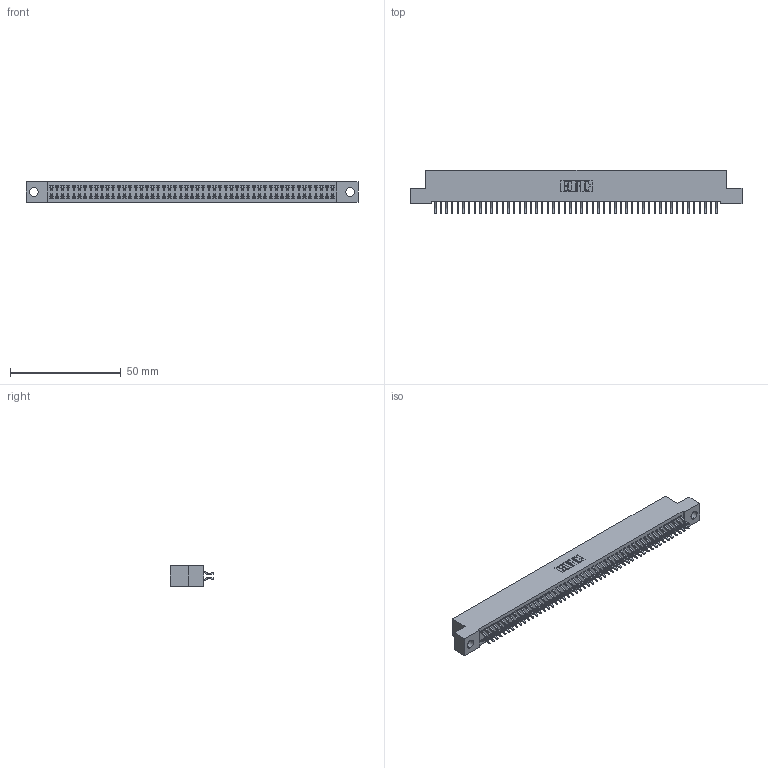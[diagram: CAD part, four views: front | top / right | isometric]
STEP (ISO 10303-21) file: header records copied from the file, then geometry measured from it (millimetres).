
FILE_DESCRIPTION (( 'STEP AP203' ), '1' );
FILE_NAME ('392-102-556-204.STEP', '2019-10-09T21:36:11', ( '' ), ( '' ), 'SwSTEP 2.0', 'SolidWorks 2016', '' );
FILE_SCHEMA (( 'CONFIG_CONTROL_DESIGN' ));
Length unit declared in the file: inch
Products named in the file (3): 342 Part_.156 TH; 345-292-001_556 Tail; 392-102-556-204
Assembly tree (103 placements, depth 2):
  392-102-556-204
    342 Part_.156 TH
    345-292-001_556 Tail  x102
Bounding box: 149.86 x 19.58 x 9.4 mm (x, y, z)
Volume: 13417.9 mm3; surface area: 21788 mm2
Topology: 103 solids, 103 shells, 6026 faces, 17945 edges, 11826 vertices
Faces by surface type: plane 4146, cylinder 1880
Entity records: 31737 total; most frequent: CARTESIAN_POINT 5262, ORIENTED_EDGE 5186, DIRECTION 4469, EDGE_CURVE 2593, VECTOR 2457, LINE 2457, VERTEX_POINT 1726, AXIS2_PLACEMENT_3D 1006
